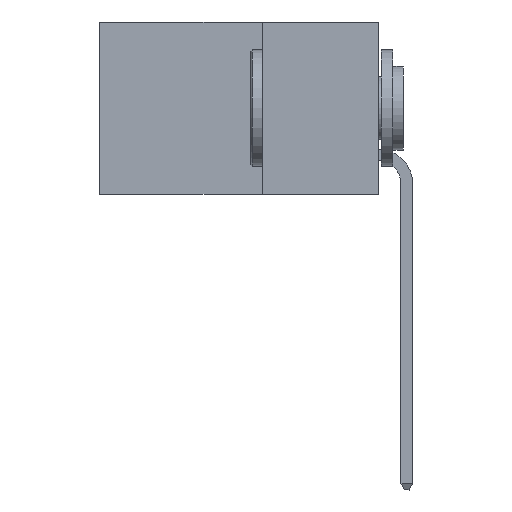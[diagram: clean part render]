
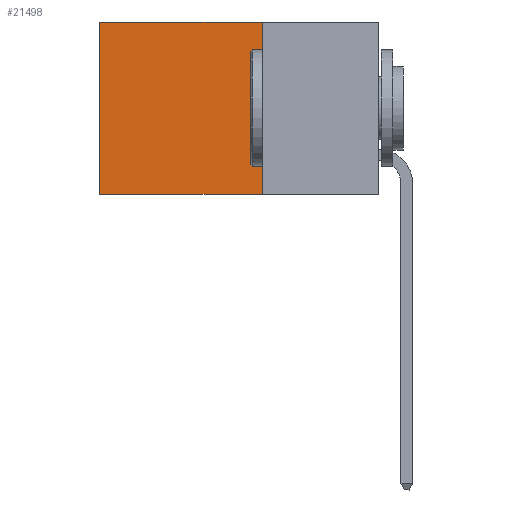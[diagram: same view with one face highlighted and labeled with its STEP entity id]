
A CAD part, left-side view. The second image highlights one B-rep face of the part: STEP entity #21498.
In plain terms, the highlighted planar face has unit normal (-1, 0, 0).
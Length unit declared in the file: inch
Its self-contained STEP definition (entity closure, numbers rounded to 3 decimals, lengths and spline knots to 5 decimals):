
#63 = VERTEX_POINT ( 'NONE', #5275 ) ;
#489 = ORIENTED_EDGE ( 'NONE', *, *, #12991, .T. ) ;
#1436 = AXIS2_PLACEMENT_3D ( 'NONE', #19309, #23598, #13775 ) ;
#1563 = PLANE ( 'NONE',  #1436 ) ;
#2110 = DIRECTION ( 'NONE',  ( 0., 0., -1. ) ) ;
#2163 = ORIENTED_EDGE ( 'NONE', *, *, #16385, .T. ) ;
#2711 = DIRECTION ( 'NONE',  ( 0., 1., 0. ) ) ;
#3654 = CARTESIAN_POINT ( 'NONE',  ( 0.2615, 0.25, 0. ) ) ;
#4697 = CARTESIAN_POINT ( 'NONE',  ( 0.2615, 0.25, 0. ) ) ;
#5275 = CARTESIAN_POINT ( 'NONE',  ( 0.2615, 0.25, -0.37 ) ) ;
#5676 = VECTOR ( 'NONE', #16147, 39.37008 ) ;
#5859 = EDGE_CURVE ( 'NONE', #12631, #63, #20509, .T. ) ;
#6603 = VECTOR ( 'NONE', #12284, 39.37008 ) ;
#6789 = CARTESIAN_POINT ( 'NONE',  ( 0.2615, 0.25, -0.37 ) ) ;
#6816 = EDGE_CURVE ( 'NONE', #63, #15160, #12803, .T. ) ;
#9682 = CARTESIAN_POINT ( 'NONE',  ( 0.2615, 0.6, 0. ) ) ;
#9823 = ORIENTED_EDGE ( 'NONE', *, *, #6816, .F. ) ;
#9971 = VECTOR ( 'NONE', #2711, 39.37008 ) ;
#10239 = CARTESIAN_POINT ( 'NONE',  ( 0.2615, 0.25, -0.37 ) ) ;
#10752 = EDGE_LOOP ( 'NONE', ( #2163, #9823, #23512, #489 ) ) ;
#11411 = FACE_OUTER_BOUND ( 'NONE', #10752, .T. ) ;
#11443 = VERTEX_POINT ( 'NONE', #9682 ) ;
#12284 = DIRECTION ( 'NONE',  ( 0., 1., 0. ) ) ;
#12631 = VERTEX_POINT ( 'NONE', #3654 ) ;
#12803 = LINE ( 'NONE', #6789, #9971 ) ;
#12991 = EDGE_CURVE ( 'NONE', #12631, #11443, #16498, .T. ) ;
#13492 = CARTESIAN_POINT ( 'NONE',  ( 0.2615, 0.6, -0.37 ) ) ;
#13775 = DIRECTION ( 'NONE',  ( 0., 0., -1. ) ) ;
#15160 = VERTEX_POINT ( 'NONE', #13492 ) ;
#16147 = DIRECTION ( 'NONE',  ( 0., 0., -1. ) ) ;
#16385 = EDGE_CURVE ( 'NONE', #11443, #15160, #22057, .T. ) ;
#16498 = LINE ( 'NONE', #4697, #6603 ) ;
#16721 = VECTOR ( 'NONE', #2110, 39.37008 ) ;
#19309 = CARTESIAN_POINT ( 'NONE',  ( 0.2615, 0.25, -0.37 ) ) ;
#20509 = LINE ( 'NONE', #10239, #16721 ) ;
#21498 = ADVANCED_FACE ( 'NONE', ( #11411 ), #1563, .F. ) ;
#22057 = LINE ( 'NONE', #23882, #5676 ) ;
#23512 = ORIENTED_EDGE ( 'NONE', *, *, #5859, .F. ) ;
#23598 = DIRECTION ( 'NONE',  ( 1., 0., 0. ) ) ;
#23882 = CARTESIAN_POINT ( 'NONE',  ( 0.2615, 0.6, -0.37 ) ) ;
